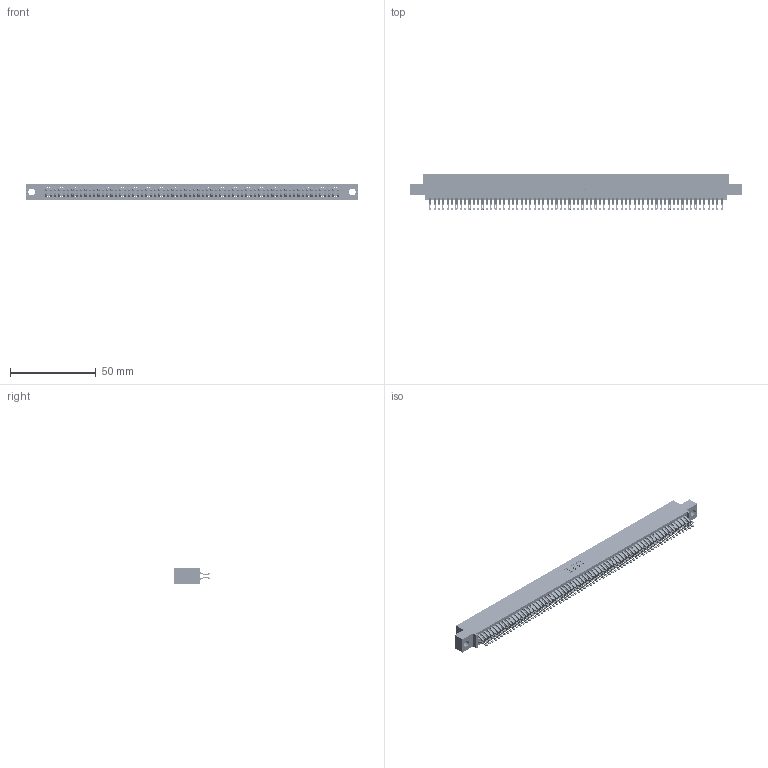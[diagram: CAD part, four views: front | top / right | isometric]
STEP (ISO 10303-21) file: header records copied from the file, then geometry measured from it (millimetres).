
FILE_DESCRIPTION (( 'STEP AP203' ), '1' );
FILE_NAME ('395-136-555-504.STEP', '2018-12-05T10:12:56', ( '' ), ( '' ), 'SwSTEP 2.0', 'SolidWorks 2016', '' );
FILE_SCHEMA (( 'CONFIG_CONTROL_DESIGN' ));
Length unit declared in the file: inch
Products named in the file (3): 395-136-555-504; 345 Part_0.110 Offset - 0.156 Dia-TH; 345-292-001_555 Tail
Assembly tree (137 placements, depth 2):
  395-136-555-504
    345 Part_0.110 Offset - 0.156 Dia-TH
    345-292-001_555 Tail  x136
Bounding box: 193.93 x 21.13 x 9.4 mm (x, y, z)
Volume: 19313.1 mm3; surface area: 30331.5 mm2
Topology: 137 solids, 137 shells, 7746 faces, 24425 edges, 16282 vertices
Faces by surface type: plane 4300, cylinder 3446
Entity records: 50315 total; most frequent: CARTESIAN_POINT 8446, ORIENTED_EDGE 8350, DIRECTION 7383, EDGE_CURVE 4175, LINE 3751, VECTOR 3751, VERTEX_POINT 2782, AXIS2_PLACEMENT_3D 1816
